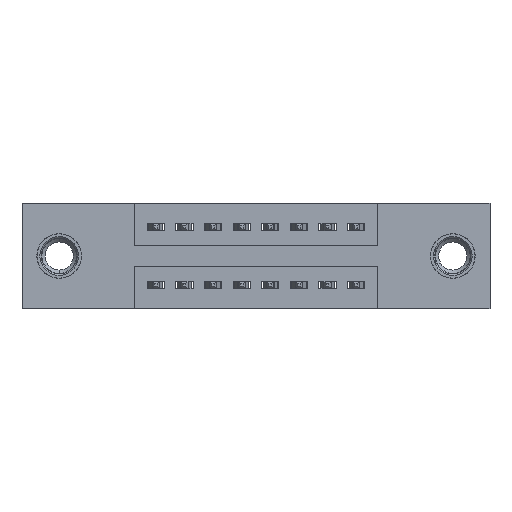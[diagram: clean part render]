
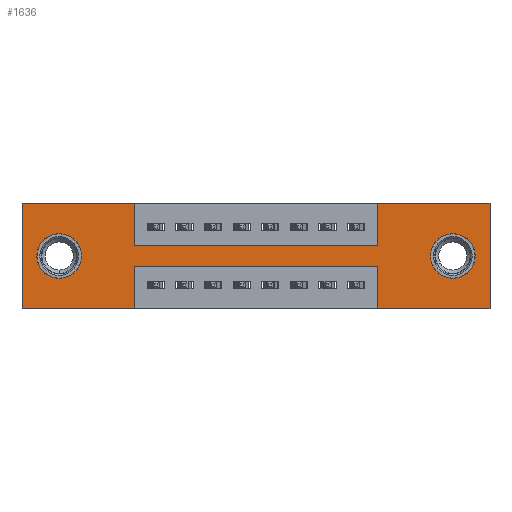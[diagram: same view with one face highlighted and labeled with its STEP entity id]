
A CAD part, front view. The second image highlights one B-rep face of the part: STEP entity #1636.
In plain terms, the highlighted planar face has unit normal (0, -1, 0).
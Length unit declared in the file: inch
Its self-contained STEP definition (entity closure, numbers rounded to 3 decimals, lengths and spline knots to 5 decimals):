
#247 = AXIS2_PLACEMENT_3D ( 'NONE', #3942, #334, #8704 ) ;
#334 = DIRECTION ( 'NONE',  ( 0., 1., 0. ) ) ;
#358 = ORIENTED_EDGE ( 'NONE', *, *, #8874, .F. ) ;
#362 = DIRECTION ( 'NONE',  ( 0., 0., -1. ) ) ;
#488 = DIRECTION ( 'NONE',  ( 0., 1., 0. ) ) ;
#581 = CARTESIAN_POINT ( 'NONE',  ( 0.3925, 0., 0. ) ) ;
#661 = ORIENTED_EDGE ( 'NONE', *, *, #11573, .F. ) ;
#797 = DIRECTION ( 'NONE',  ( 0., 0., -1. ) ) ;
#839 = CARTESIAN_POINT ( 'NONE',  ( 0., 0., -0.37 ) ) ;
#870 = DIRECTION ( 'NONE',  ( 1., 0., 0. ) ) ;
#1049 = CARTESIAN_POINT ( 'NONE',  ( 0.3925, 0., -0.37 ) ) ;
#1100 = CARTESIAN_POINT ( 'NONE',  ( 1.2425, 0., 0. ) ) ;
#1255 = DIRECTION ( 'NONE',  ( 0., 0., 1. ) ) ;
#1274 = ORIENTED_EDGE ( 'NONE', *, *, #2866, .F. ) ;
#1322 = CIRCLE ( 'NONE', #4395, 0.078 ) ;
#1368 = CARTESIAN_POINT ( 'NONE',  ( 0.3925, 0., -0.37 ) ) ;
#1438 = EDGE_CURVE ( 'NONE', #6066, #8206, #4165, .T. ) ;
#1505 = EDGE_CURVE ( 'NONE', #8206, #2194, #8786, .T. ) ;
#1580 = VECTOR ( 'NONE', #797, 39.37008 ) ;
#1610 = LINE ( 'NONE', #1852, #11270 ) ;
#1636 = ADVANCED_FACE ( 'NONE', ( #9980, #11141, #10702 ), #9591, .T. ) ;
#1705 = AXIS2_PLACEMENT_3D ( 'NONE', #11453, #9633, #362 ) ;
#1741 = VERTEX_POINT ( 'NONE', #6367 ) ;
#1852 = CARTESIAN_POINT ( 'NONE',  ( 1.2425, 0., -0.37 ) ) ;
#1858 = EDGE_CURVE ( 'NONE', #10796, #8619, #7008, .T. ) ;
#1876 = CARTESIAN_POINT ( 'NONE',  ( 0.13, 0., -0.185 ) ) ;
#1981 = EDGE_CURVE ( 'NONE', #9061, #7783, #2082, .T. ) ;
#2081 = VECTOR ( 'NONE', #8409, 39.37008 ) ;
#2082 = LINE ( 'NONE', #3191, #2977 ) ;
#2194 = VERTEX_POINT ( 'NONE', #3375 ) ;
#2208 = ORIENTED_EDGE ( 'NONE', *, *, #1438, .F. ) ;
#2225 = CARTESIAN_POINT ( 'NONE',  ( 0.3925, 0., -0.15 ) ) ;
#2301 = EDGE_CURVE ( 'NONE', #11989, #6574, #2814, .T. ) ;
#2304 = VERTEX_POINT ( 'NONE', #8405 ) ;
#2318 = CIRCLE ( 'NONE', #7842, 0.078 ) ;
#2594 = EDGE_CURVE ( 'NONE', #2304, #11301, #1322, .T. ) ;
#2619 = CARTESIAN_POINT ( 'NONE',  ( 1.505, 0., -0.107 ) ) ;
#2647 = CARTESIAN_POINT ( 'NONE',  ( 1.635, 0., 0. ) ) ;
#2814 = LINE ( 'NONE', #6449, #9060 ) ;
#2846 = VECTOR ( 'NONE', #7093, 39.37008 ) ;
#2864 = CIRCLE ( 'NONE', #3145, 0.078 ) ;
#2866 = EDGE_CURVE ( 'NONE', #11570, #9927, #1610, .T. ) ;
#2977 = VECTOR ( 'NONE', #6024, 39.37008 ) ;
#3075 = CARTESIAN_POINT ( 'NONE',  ( 1.2425, 0., -0.22 ) ) ;
#3145 = AXIS2_PLACEMENT_3D ( 'NONE', #4939, #5851, #7697 ) ;
#3191 = CARTESIAN_POINT ( 'NONE',  ( 0.3925, 0., -0.15 ) ) ;
#3375 = CARTESIAN_POINT ( 'NONE',  ( 1.635, 0., -0.37 ) ) ;
#3453 = EDGE_CURVE ( 'NONE', #6462, #9018, #5983, .T. ) ;
#3563 = CARTESIAN_POINT ( 'NONE',  ( 0.3925, 0., 0. ) ) ;
#3671 = EDGE_LOOP ( 'NONE', ( #6842, #8494 ) ) ;
#3743 = CARTESIAN_POINT ( 'NONE',  ( 1.635, 0., 0. ) ) ;
#3775 = CARTESIAN_POINT ( 'NONE',  ( 1.505, 0., -0.263 ) ) ;
#3906 = EDGE_LOOP ( 'NONE', ( #9349, #5624 ) ) ;
#3942 = CARTESIAN_POINT ( 'NONE',  ( 1.505, 0., -0.185 ) ) ;
#3974 = EDGE_CURVE ( 'NONE', #1741, #6462, #10060, .T. ) ;
#4088 = LINE ( 'NONE', #8620, #11056 ) ;
#4165 = LINE ( 'NONE', #9903, #2846 ) ;
#4395 = AXIS2_PLACEMENT_3D ( 'NONE', #10668, #488, #6189 ) ;
#4430 = CARTESIAN_POINT ( 'NONE',  ( 0.3925, 0., -0.22 ) ) ;
#4606 = ORIENTED_EDGE ( 'NONE', *, *, #3974, .F. ) ;
#4623 = LINE ( 'NONE', #1100, #9558 ) ;
#4939 = CARTESIAN_POINT ( 'NONE',  ( 1.505, 0., -0.185 ) ) ;
#4986 = ORIENTED_EDGE ( 'NONE', *, *, #1981, .F. ) ;
#5144 = ORIENTED_EDGE ( 'NONE', *, *, #2301, .F. ) ;
#5624 = ORIENTED_EDGE ( 'NONE', *, *, #10626, .T. ) ;
#5851 = DIRECTION ( 'NONE',  ( 0., 1., 0. ) ) ;
#5942 = CARTESIAN_POINT ( 'NONE',  ( 0., 0., 0. ) ) ;
#5977 = ORIENTED_EDGE ( 'NONE', *, *, #6265, .F. ) ;
#5983 = LINE ( 'NONE', #10650, #9171 ) ;
#6024 = DIRECTION ( 'NONE',  ( 1., 0., 0. ) ) ;
#6066 = VERTEX_POINT ( 'NONE', #11264 ) ;
#6189 = DIRECTION ( 'NONE',  ( 0., 0., 1. ) ) ;
#6222 = ORIENTED_EDGE ( 'NONE', *, *, #10047, .F. ) ;
#6265 = EDGE_CURVE ( 'NONE', #2194, #11570, #6872, .T. ) ;
#6367 = CARTESIAN_POINT ( 'NONE',  ( 0.3925, 0., -0.22 ) ) ;
#6449 = CARTESIAN_POINT ( 'NONE',  ( 0., 0., 0. ) ) ;
#6462 = VERTEX_POINT ( 'NONE', #1049 ) ;
#6574 = VERTEX_POINT ( 'NONE', #581 ) ;
#6810 = CARTESIAN_POINT ( 'NONE',  ( 1.2425, 0., -0.15 ) ) ;
#6842 = ORIENTED_EDGE ( 'NONE', *, *, #7906, .T. ) ;
#6872 = LINE ( 'NONE', #839, #2081 ) ;
#7008 = CIRCLE ( 'NONE', #247, 0.078 ) ;
#7093 = DIRECTION ( 'NONE',  ( 1., 0., 0. ) ) ;
#7233 = ORIENTED_EDGE ( 'NONE', *, *, #3453, .F. ) ;
#7344 = DIRECTION ( 'NONE',  ( 0., 0., -1. ) ) ;
#7368 = DIRECTION ( 'NONE',  ( 0., 0., 1. ) ) ;
#7697 = DIRECTION ( 'NONE',  ( 0., 0., -1. ) ) ;
#7783 = VERTEX_POINT ( 'NONE', #6810 ) ;
#7842 = AXIS2_PLACEMENT_3D ( 'NONE', #1876, #9420, #7368 ) ;
#7906 = EDGE_CURVE ( 'NONE', #11301, #2304, #2318, .T. ) ;
#8206 = VERTEX_POINT ( 'NONE', #3743 ) ;
#8405 = CARTESIAN_POINT ( 'NONE',  ( 0.13, 0., -0.263 ) ) ;
#8409 = DIRECTION ( 'NONE',  ( -1., 0., 0. ) ) ;
#8494 = ORIENTED_EDGE ( 'NONE', *, *, #2594, .T. ) ;
#8619 = VERTEX_POINT ( 'NONE', #3775 ) ;
#8620 = CARTESIAN_POINT ( 'NONE',  ( 0., 0., 0. ) ) ;
#8704 = DIRECTION ( 'NONE',  ( 0., 0., -1. ) ) ;
#8786 = LINE ( 'NONE', #2647, #9387 ) ;
#8789 = VECTOR ( 'NONE', #9145, 39.37008 ) ;
#8798 = LINE ( 'NONE', #4430, #11766 ) ;
#8874 = EDGE_CURVE ( 'NONE', #9018, #11989, #4088, .T. ) ;
#9018 = VERTEX_POINT ( 'NONE', #11504 ) ;
#9060 = VECTOR ( 'NONE', #870, 39.37008 ) ;
#9061 = VERTEX_POINT ( 'NONE', #2225 ) ;
#9086 = LINE ( 'NONE', #3563, #8789 ) ;
#9145 = DIRECTION ( 'NONE',  ( 0., 0., -1. ) ) ;
#9171 = VECTOR ( 'NONE', #9709, 39.37008 ) ;
#9349 = ORIENTED_EDGE ( 'NONE', *, *, #1858, .T. ) ;
#9387 = VECTOR ( 'NONE', #7344, 39.37008 ) ;
#9420 = DIRECTION ( 'NONE',  ( 0., 1., 0. ) ) ;
#9484 = DIRECTION ( 'NONE',  ( 0., 0., 1. ) ) ;
#9558 = VECTOR ( 'NONE', #1255, 39.37008 ) ;
#9563 = ORIENTED_EDGE ( 'NONE', *, *, #10909, .F. ) ;
#9591 = PLANE ( 'NONE',  #1705 ) ;
#9633 = DIRECTION ( 'NONE',  ( 0., -1., 0. ) ) ;
#9709 = DIRECTION ( 'NONE',  ( -1., 0., 0. ) ) ;
#9903 = CARTESIAN_POINT ( 'NONE',  ( 0., 0., 0. ) ) ;
#9927 = VERTEX_POINT ( 'NONE', #3075 ) ;
#9980 = FACE_BOUND ( 'NONE', #3906, .T. ) ;
#10047 = EDGE_CURVE ( 'NONE', #7783, #6066, #4623, .T. ) ;
#10060 = LINE ( 'NONE', #1368, #1580 ) ;
#10071 = ORIENTED_EDGE ( 'NONE', *, *, #1505, .F. ) ;
#10310 = DIRECTION ( 'NONE',  ( 0., 0., 1. ) ) ;
#10562 = CARTESIAN_POINT ( 'NONE',  ( 0.13, 0., -0.107 ) ) ;
#10626 = EDGE_CURVE ( 'NONE', #8619, #10796, #2864, .T. ) ;
#10650 = CARTESIAN_POINT ( 'NONE',  ( 0., 0., -0.37 ) ) ;
#10668 = CARTESIAN_POINT ( 'NONE',  ( 0.13, 0., -0.185 ) ) ;
#10702 = FACE_OUTER_BOUND ( 'NONE', #11688, .T. ) ;
#10796 = VERTEX_POINT ( 'NONE', #2619 ) ;
#10909 = EDGE_CURVE ( 'NONE', #9927, #1741, #8798, .T. ) ;
#10931 = DIRECTION ( 'NONE',  ( -1., 0., 0. ) ) ;
#11056 = VECTOR ( 'NONE', #9484, 39.37008 ) ;
#11141 = FACE_BOUND ( 'NONE', #3671, .T. ) ;
#11264 = CARTESIAN_POINT ( 'NONE',  ( 1.2425, 0., 0. ) ) ;
#11270 = VECTOR ( 'NONE', #10310, 39.37008 ) ;
#11301 = VERTEX_POINT ( 'NONE', #10562 ) ;
#11453 = CARTESIAN_POINT ( 'NONE',  ( 0., 0., -0.37 ) ) ;
#11504 = CARTESIAN_POINT ( 'NONE',  ( 0., 0., -0.37 ) ) ;
#11570 = VERTEX_POINT ( 'NONE', #11950 ) ;
#11573 = EDGE_CURVE ( 'NONE', #6574, #9061, #9086, .T. ) ;
#11688 = EDGE_LOOP ( 'NONE', ( #4606, #9563, #1274, #5977, #10071, #2208, #6222, #4986, #661, #5144, #358, #7233 ) ) ;
#11766 = VECTOR ( 'NONE', #10931, 39.37008 ) ;
#11950 = CARTESIAN_POINT ( 'NONE',  ( 1.2425, 0., -0.37 ) ) ;
#11989 = VERTEX_POINT ( 'NONE', #5942 ) ;
